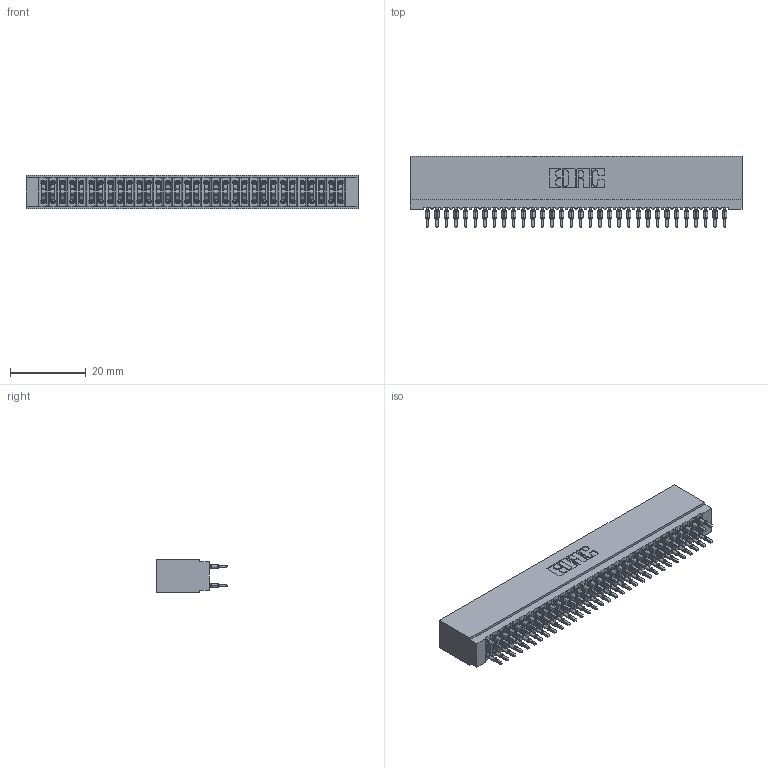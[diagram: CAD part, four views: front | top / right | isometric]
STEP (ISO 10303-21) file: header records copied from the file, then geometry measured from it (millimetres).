
FILE_DESCRIPTION (( 'STEP AP203' ), '1' );
FILE_NAME ('725-064-560-201.STEP', '2026-02-24T18:23:59', ( '' ), ( '' ), 'SwSTEP 2.0', 'SolidWorks 2023', '' );
FILE_SCHEMA (( 'CONFIG_CONTROL_DESIGN' ));
Length unit declared in the file: millimetre
Products named in the file (3): 725-064-560-201; 745-292-001_560; 725 Part_Insulator Option - 01
Assembly tree (65 placements, depth 2):
  725-064-560-201
    725 Part_Insulator Option - 01
    745-292-001_560  x64
Bounding box: 87.88 x 18.8 x 8.89 mm (x, y, z)
Volume: 7256.1 mm3; surface area: 16121 mm2
Topology: 65 solids, 65 shells, 6399 faces, 17502 edges, 11112 vertices
Faces by surface type: plane 3319, cylinder 1416, bspline 1280, torus 384
Entity records: 55525 total; most frequent: CARTESIAN_POINT 10137, ORIENTED_EDGE 9552, DIRECTION 8360, EDGE_CURVE 4776, VECTOR 4394, LINE 4394, VERTEX_POINT 3048, AXIS2_PLACEMENT_3D 1983
